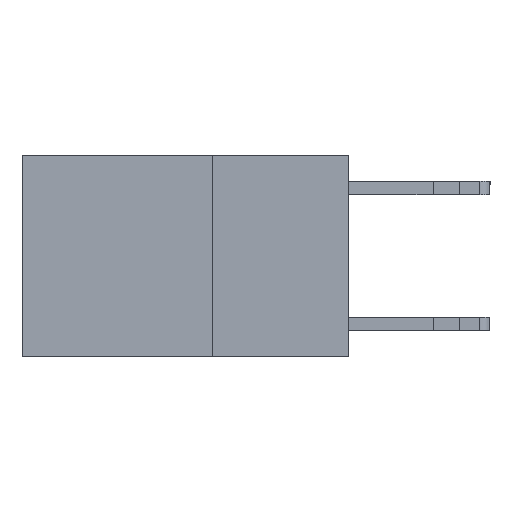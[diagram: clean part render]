
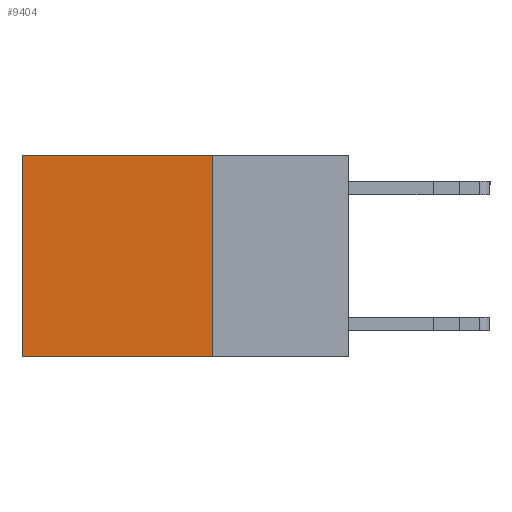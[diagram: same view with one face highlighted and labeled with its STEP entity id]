
A CAD part, left-side view. The second image highlights one B-rep face of the part: STEP entity #9404.
In plain terms, the highlighted planar face has unit normal (-1, 0, 0).
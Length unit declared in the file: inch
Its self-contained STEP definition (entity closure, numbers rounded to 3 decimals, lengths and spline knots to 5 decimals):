
#196 = VERTEX_POINT ( 'NONE', #16398 ) ;
#2039 = ORIENTED_EDGE ( 'NONE', *, *, #14872, .T. ) ;
#3818 = VECTOR ( 'NONE', #24100, 39.37008 ) ;
#4351 = EDGE_CURVE ( 'NONE', #22386, #4946, #12676, .T. ) ;
#4946 = VERTEX_POINT ( 'NONE', #15695 ) ;
#5196 = DIRECTION ( 'NONE',  ( 1., 0., 0. ) ) ;
#5652 = ORIENTED_EDGE ( 'NONE', *, *, #16015, .T. ) ;
#5747 = LINE ( 'NONE', #22354, #3818 ) ;
#6123 = CARTESIAN_POINT ( 'NONE',  ( 0.2625, 0.6, 0. ) ) ;
#7441 = CARTESIAN_POINT ( 'NONE',  ( 0.2625, 0.25, -0.37 ) ) ;
#7860 = VERTEX_POINT ( 'NONE', #6123 ) ;
#8217 = DIRECTION ( 'NONE',  ( 0., 0., -1. ) ) ;
#8637 = VECTOR ( 'NONE', #18824, 39.37008 ) ;
#9227 = DIRECTION ( 'NONE',  ( 0., 0., -1. ) ) ;
#9404 = ADVANCED_FACE ( 'NONE', ( #21269 ), #19527, .F. ) ;
#10106 = EDGE_LOOP ( 'NONE', ( #5652, #20129, #17572, #2039 ) ) ;
#10375 = CARTESIAN_POINT ( 'NONE',  ( 0.2625, 0.25, 0. ) ) ;
#12676 = LINE ( 'NONE', #20829, #8637 ) ;
#13093 = CARTESIAN_POINT ( 'NONE',  ( 0.2625, 0.6, 0. ) ) ;
#14872 = EDGE_CURVE ( 'NONE', #196, #7860, #5747, .T. ) ;
#15695 = CARTESIAN_POINT ( 'NONE',  ( 0.2625, 0.6, -0.37 ) ) ;
#16015 = EDGE_CURVE ( 'NONE', #7860, #4946, #22757, .T. ) ;
#16084 = AXIS2_PLACEMENT_3D ( 'NONE', #21537, #5196, #9227 ) ;
#16176 = VECTOR ( 'NONE', #20728, 39.37008 ) ;
#16398 = CARTESIAN_POINT ( 'NONE',  ( 0.2625, 0.25, 0. ) ) ;
#17572 = ORIENTED_EDGE ( 'NONE', *, *, #19498, .F. ) ;
#18824 = DIRECTION ( 'NONE',  ( 0., 1., 0. ) ) ;
#19498 = EDGE_CURVE ( 'NONE', #196, #22386, #20526, .T. ) ;
#19527 = PLANE ( 'NONE',  #16084 ) ;
#20129 = ORIENTED_EDGE ( 'NONE', *, *, #4351, .F. ) ;
#20526 = LINE ( 'NONE', #10375, #21857 ) ;
#20728 = DIRECTION ( 'NONE',  ( 0., 0., -1. ) ) ;
#20829 = CARTESIAN_POINT ( 'NONE',  ( 0.2625, 0.25, -0.37 ) ) ;
#21269 = FACE_OUTER_BOUND ( 'NONE', #10106, .T. ) ;
#21537 = CARTESIAN_POINT ( 'NONE',  ( 0.2625, 0.25, 0. ) ) ;
#21857 = VECTOR ( 'NONE', #8217, 39.37008 ) ;
#22354 = CARTESIAN_POINT ( 'NONE',  ( 0.2625, 0.25, 0. ) ) ;
#22386 = VERTEX_POINT ( 'NONE', #7441 ) ;
#22757 = LINE ( 'NONE', #13093, #16176 ) ;
#24100 = DIRECTION ( 'NONE',  ( 0., 1., 0. ) ) ;
